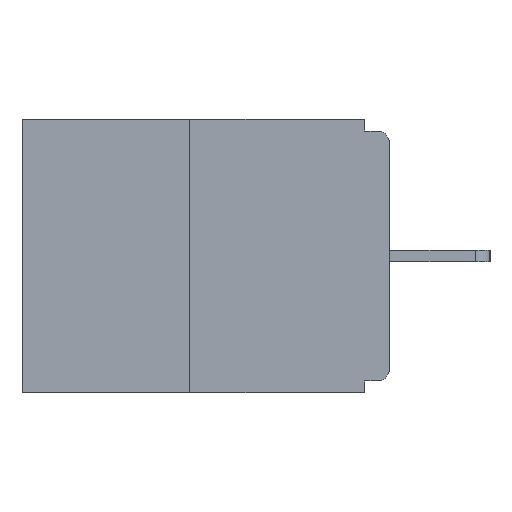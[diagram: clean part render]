
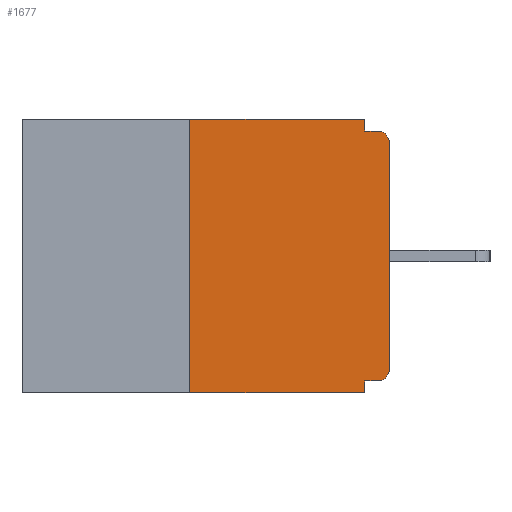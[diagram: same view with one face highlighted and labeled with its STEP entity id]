
A CAD part, left-side view. The second image highlights one B-rep face of the part: STEP entity #1677.
In plain terms, the highlighted planar face has unit normal (-1, 0, 0).
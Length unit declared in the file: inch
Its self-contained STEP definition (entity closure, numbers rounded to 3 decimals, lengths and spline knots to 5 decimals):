
#56 = ORIENTED_EDGE ( 'NONE', *, *, #13079, .T. ) ;
#352 = ORIENTED_EDGE ( 'NONE', *, *, #5008, .F. ) ;
#638 = AXIS2_PLACEMENT_3D ( 'NONE', #13211, #4932, #5860 ) ;
#729 = LINE ( 'NONE', #4089, #11823 ) ;
#1007 = ORIENTED_EDGE ( 'NONE', *, *, #8460, .F. ) ;
#1121 = DIRECTION ( 'NONE',  ( 0., 0., -1. ) ) ;
#1307 = LINE ( 'NONE', #11826, #4190 ) ;
#1384 = LINE ( 'NONE', #5670, #1891 ) ;
#1521 = CARTESIAN_POINT ( 'NONE',  ( 0., 0.031, -0.343 ) ) ;
#1608 = ORIENTED_EDGE ( 'NONE', *, *, #9251, .F. ) ;
#1677 = ADVANCED_FACE ( 'NONE', ( #9022 ), #2701, .F. ) ;
#1891 = VECTOR ( 'NONE', #9954, 39.37008 ) ;
#1944 = VECTOR ( 'NONE', #9618, 39.37008 ) ;
#2008 = ORIENTED_EDGE ( 'NONE', *, *, #13532, .F. ) ;
#2018 = DIRECTION ( 'NONE',  ( 0., 0., 1. ) ) ;
#2451 = VECTOR ( 'NONE', #2018, 39.37008 ) ;
#2701 = PLANE ( 'NONE',  #638 ) ;
#3073 = CARTESIAN_POINT ( 'NONE',  ( 0., 0., -0.03 ) ) ;
#3156 = EDGE_CURVE ( 'NONE', #13667, #12984, #9866, .T. ) ;
#3208 = EDGE_LOOP ( 'NONE', ( #7384, #1608, #8091, #352, #2008, #5824, #56, #5209, #1007, #8433 ) ) ;
#3280 = CARTESIAN_POINT ( 'NONE',  ( 0., 0.015, -0.313 ) ) ;
#3281 = EDGE_CURVE ( 'NONE', #5180, #13134, #4330, .T. ) ;
#3413 = LINE ( 'NONE', #13020, #1944 ) ;
#3959 = VERTEX_POINT ( 'NONE', #13682 ) ;
#3963 = CARTESIAN_POINT ( 'NONE',  ( 0., 0.25, -0.343 ) ) ;
#4089 = CARTESIAN_POINT ( 'NONE',  ( 0., 0., -0.015 ) ) ;
#4121 = VECTOR ( 'NONE', #11056, 39.37008 ) ;
#4190 = VECTOR ( 'NONE', #7440, 39.37008 ) ;
#4330 = LINE ( 'NONE', #8634, #9423 ) ;
#4507 = VERTEX_POINT ( 'NONE', #5466 ) ;
#4619 = DIRECTION ( 'NONE',  ( 0., 0., -1. ) ) ;
#4932 = DIRECTION ( 'NONE',  ( 1., 0., 0. ) ) ;
#5008 = EDGE_CURVE ( 'NONE', #4507, #13134, #7786, .T. ) ;
#5055 = DIRECTION ( 'NONE',  ( 0., -1., 0. ) ) ;
#5073 = EDGE_CURVE ( 'NONE', #5335, #11462, #1384, .T. ) ;
#5180 = VERTEX_POINT ( 'NONE', #3963 ) ;
#5209 = ORIENTED_EDGE ( 'NONE', *, *, #9090, .T. ) ;
#5303 = VERTEX_POINT ( 'NONE', #12656 ) ;
#5335 = VERTEX_POINT ( 'NONE', #10880 ) ;
#5466 = CARTESIAN_POINT ( 'NONE',  ( 0., 0.031, -0.328 ) ) ;
#5534 = CARTESIAN_POINT ( 'NONE',  ( 0., 0.031, -0.343 ) ) ;
#5670 = CARTESIAN_POINT ( 'NONE',  ( 0., 0.031, 0. ) ) ;
#5824 = ORIENTED_EDGE ( 'NONE', *, *, #3156, .T. ) ;
#5860 = DIRECTION ( 'NONE',  ( 0., 0., -1. ) ) ;
#6325 = CARTESIAN_POINT ( 'NONE',  ( 0., 0., -0.313 ) ) ;
#6818 = CARTESIAN_POINT ( 'NONE',  ( 0., 0.015, -0.03 ) ) ;
#7357 = LINE ( 'NONE', #8352, #2451 ) ;
#7384 = ORIENTED_EDGE ( 'NONE', *, *, #13775, .F. ) ;
#7440 = DIRECTION ( 'NONE',  ( 0., 1., 0. ) ) ;
#7544 = VERTEX_POINT ( 'NONE', #3073 ) ;
#7605 = AXIS2_PLACEMENT_3D ( 'NONE', #6818, #10866, #4619 ) ;
#7786 = LINE ( 'NONE', #1521, #4121 ) ;
#8091 = ORIENTED_EDGE ( 'NONE', *, *, #3281, .T. ) ;
#8251 = VECTOR ( 'NONE', #5055, 39.37008 ) ;
#8320 = CARTESIAN_POINT ( 'NONE',  ( 0., 0.46, 0. ) ) ;
#8352 = CARTESIAN_POINT ( 'NONE',  ( 0., 0.25, 0. ) ) ;
#8433 = ORIENTED_EDGE ( 'NONE', *, *, #5073, .F. ) ;
#8460 = EDGE_CURVE ( 'NONE', #11462, #3959, #729, .T. ) ;
#8634 = CARTESIAN_POINT ( 'NONE',  ( 0., 0.46, -0.343 ) ) ;
#9022 = FACE_OUTER_BOUND ( 'NONE', #3208, .T. ) ;
#9090 = EDGE_CURVE ( 'NONE', #7544, #3959, #12954, .T. ) ;
#9251 = EDGE_CURVE ( 'NONE', #5180, #5303, #7357, .T. ) ;
#9356 = LINE ( 'NONE', #8320, #8251 ) ;
#9423 = VECTOR ( 'NONE', #12886, 39.37008 ) ;
#9618 = DIRECTION ( 'NONE',  ( 0., 0., 1. ) ) ;
#9866 = CIRCLE ( 'NONE', #11650, 0.015 ) ;
#9954 = DIRECTION ( 'NONE',  ( 0., 0., -1. ) ) ;
#10796 = DIRECTION ( 'NONE',  ( -1., 0., 0. ) ) ;
#10866 = DIRECTION ( 'NONE',  ( -1., 0., 0. ) ) ;
#10880 = CARTESIAN_POINT ( 'NONE',  ( 0., 0.031, 0. ) ) ;
#11056 = DIRECTION ( 'NONE',  ( 0., 0., -1. ) ) ;
#11462 = VERTEX_POINT ( 'NONE', #12896 ) ;
#11650 = AXIS2_PLACEMENT_3D ( 'NONE', #3280, #10796, #1121 ) ;
#11823 = VECTOR ( 'NONE', #12508, 39.37008 ) ;
#11826 = CARTESIAN_POINT ( 'NONE',  ( 0., 0., -0.328 ) ) ;
#12508 = DIRECTION ( 'NONE',  ( 0., -1., 0. ) ) ;
#12656 = CARTESIAN_POINT ( 'NONE',  ( 0., 0.25, 0. ) ) ;
#12886 = DIRECTION ( 'NONE',  ( 0., -1., 0. ) ) ;
#12896 = CARTESIAN_POINT ( 'NONE',  ( 0., 0.031, -0.015 ) ) ;
#12954 = CIRCLE ( 'NONE', #7605, 0.015 ) ;
#12984 = VERTEX_POINT ( 'NONE', #6325 ) ;
#13020 = CARTESIAN_POINT ( 'NONE',  ( 0., 0., 0. ) ) ;
#13079 = EDGE_CURVE ( 'NONE', #12984, #7544, #3413, .T. ) ;
#13134 = VERTEX_POINT ( 'NONE', #5534 ) ;
#13211 = CARTESIAN_POINT ( 'NONE',  ( 0., 0.46, 0. ) ) ;
#13532 = EDGE_CURVE ( 'NONE', #13667, #4507, #1307, .T. ) ;
#13533 = CARTESIAN_POINT ( 'NONE',  ( 0., 0.015, -0.328 ) ) ;
#13667 = VERTEX_POINT ( 'NONE', #13533 ) ;
#13682 = CARTESIAN_POINT ( 'NONE',  ( 0., 0.015, -0.015 ) ) ;
#13775 = EDGE_CURVE ( 'NONE', #5303, #5335, #9356, .T. ) ;
